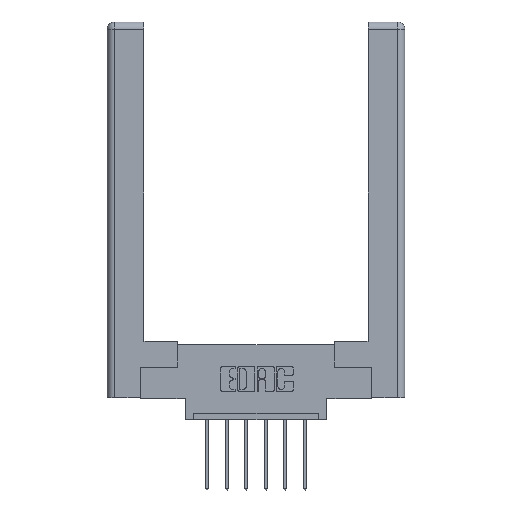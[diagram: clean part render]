
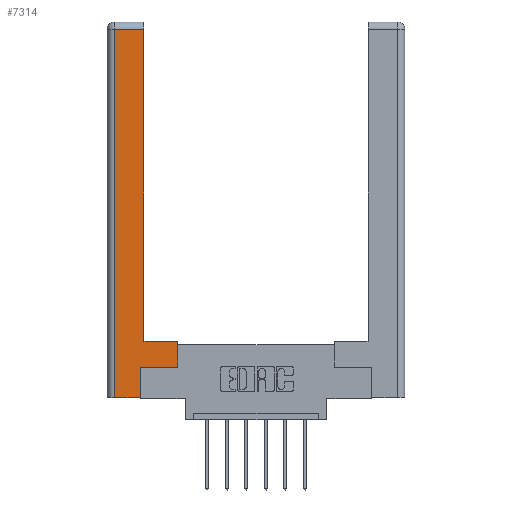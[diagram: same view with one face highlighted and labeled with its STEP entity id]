
A CAD part, top view. The second image highlights one B-rep face of the part: STEP entity #7314.
In plain terms, the highlighted planar face has unit normal (0, 0, 1).
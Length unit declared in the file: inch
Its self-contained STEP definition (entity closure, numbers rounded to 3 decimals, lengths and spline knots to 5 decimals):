
#93 = VECTOR ( 'NONE', #2105, 39.37008 ) ;
#392 = LINE ( 'NONE', #5843, #8719 ) ;
#776 = CARTESIAN_POINT ( 'NONE',  ( 0.265, 0., 0. ) ) ;
#900 = EDGE_CURVE ( 'NONE', #10897, #3169, #6829, .T. ) ;
#1043 = VERTEX_POINT ( 'NONE', #1053 ) ;
#1053 = CARTESIAN_POINT ( 'NONE',  ( 0.295, 0.45, 0. ) ) ;
#1106 = CARTESIAN_POINT ( 'NONE',  ( 0.295, 0.45, 0. ) ) ;
#1300 = LINE ( 'NONE', #4418, #10371 ) ;
#1707 = DIRECTION ( 'NONE',  ( 1., 0., 0. ) ) ;
#1950 = EDGE_CURVE ( 'NONE', #5651, #7742, #2416, .T. ) ;
#2014 = EDGE_LOOP ( 'NONE', ( #5442, #11224, #11188, #4874, #5051, #2156, #10419, #2401 ) ) ;
#2045 = DIRECTION ( 'NONE',  ( -1., 0., 0. ) ) ;
#2065 = CARTESIAN_POINT ( 'NONE',  ( 0.295, 3., 0. ) ) ;
#2073 = CARTESIAN_POINT ( 'NONE',  ( 0.565, 0.45, 0. ) ) ;
#2105 = DIRECTION ( 'NONE',  ( 0., 1., 0. ) ) ;
#2119 = AXIS2_PLACEMENT_3D ( 'NONE', #5973, #4154, #7884 ) ;
#2127 = EDGE_CURVE ( 'NONE', #2699, #1043, #5399, .T. ) ;
#2156 = ORIENTED_EDGE ( 'NONE', *, *, #8149, .T. ) ;
#2305 = VECTOR ( 'NONE', #10930, 39.37008 ) ;
#2401 = ORIENTED_EDGE ( 'NONE', *, *, #2127, .T. ) ;
#2416 = LINE ( 'NONE', #8247, #8305 ) ;
#2514 = VECTOR ( 'NONE', #1707, 39.37008 ) ;
#2685 = EDGE_CURVE ( 'NONE', #9537, #2699, #392, .T. ) ;
#2699 = VERTEX_POINT ( 'NONE', #2073 ) ;
#3102 = CARTESIAN_POINT ( 'NONE',  ( 0.265, 0., 0. ) ) ;
#3169 = VERTEX_POINT ( 'NONE', #3102 ) ;
#3200 = PLANE ( 'NONE',  #2119 ) ;
#3657 = CARTESIAN_POINT ( 'NONE',  ( 0.565, 0.245, 0. ) ) ;
#4154 = DIRECTION ( 'NONE',  ( 0., 0., -1. ) ) ;
#4418 = CARTESIAN_POINT ( 'NONE',  ( 0.0615, 0., 0. ) ) ;
#4874 = ORIENTED_EDGE ( 'NONE', *, *, #900, .T. ) ;
#5051 = ORIENTED_EDGE ( 'NONE', *, *, #8504, .T. ) ;
#5255 = FACE_OUTER_BOUND ( 'NONE', #2014, .T. ) ;
#5277 = VECTOR ( 'NONE', #7592, 39.37008 ) ;
#5399 = LINE ( 'NONE', #1106, #5695 ) ;
#5442 = ORIENTED_EDGE ( 'NONE', *, *, #10833, .T. ) ;
#5651 = VERTEX_POINT ( 'NONE', #9942 ) ;
#5695 = VECTOR ( 'NONE', #2045, 39.37008 ) ;
#5843 = CARTESIAN_POINT ( 'NONE',  ( 0.565, 0.45, 0. ) ) ;
#5973 = CARTESIAN_POINT ( 'NONE',  ( 0., 0., 0. ) ) ;
#6829 = LINE ( 'NONE', #776, #2514 ) ;
#6848 = CARTESIAN_POINT ( 'NONE',  ( 0.265, 0.245, 0. ) ) ;
#7193 = EDGE_CURVE ( 'NONE', #7742, #10897, #1300, .T. ) ;
#7253 = LINE ( 'NONE', #2065, #93 ) ;
#7309 = CARTESIAN_POINT ( 'NONE',  ( 0.565, 0.245, 0. ) ) ;
#7314 = ADVANCED_FACE ( 'NONE', ( #5255 ), #3200, .F. ) ;
#7465 = VERTEX_POINT ( 'NONE', #10876 ) ;
#7592 = DIRECTION ( 'NONE',  ( 0., 1., 0. ) ) ;
#7691 = CARTESIAN_POINT ( 'NONE',  ( 0.0615, 2.94, 0. ) ) ;
#7742 = VERTEX_POINT ( 'NONE', #7691 ) ;
#7884 = DIRECTION ( 'NONE',  ( -1., 0., 0. ) ) ;
#8065 = LINE ( 'NONE', #3657, #2305 ) ;
#8149 = EDGE_CURVE ( 'NONE', #7465, #9537, #8065, .T. ) ;
#8247 = CARTESIAN_POINT ( 'NONE',  ( 0.0615, 2.94, 0. ) ) ;
#8305 = VECTOR ( 'NONE', #11902, 39.37008 ) ;
#8332 = LINE ( 'NONE', #6848, #5277 ) ;
#8504 = EDGE_CURVE ( 'NONE', #3169, #7465, #8332, .T. ) ;
#8719 = VECTOR ( 'NONE', #11454, 39.37008 ) ;
#9537 = VERTEX_POINT ( 'NONE', #7309 ) ;
#9757 = CARTESIAN_POINT ( 'NONE',  ( 0.0615, 0., 0. ) ) ;
#9942 = CARTESIAN_POINT ( 'NONE',  ( 0.295, 2.94, 0. ) ) ;
#10371 = VECTOR ( 'NONE', #10798, 39.37008 ) ;
#10419 = ORIENTED_EDGE ( 'NONE', *, *, #2685, .T. ) ;
#10798 = DIRECTION ( 'NONE',  ( 0., -1., 0. ) ) ;
#10833 = EDGE_CURVE ( 'NONE', #1043, #5651, #7253, .T. ) ;
#10876 = CARTESIAN_POINT ( 'NONE',  ( 0.265, 0.245, 0. ) ) ;
#10897 = VERTEX_POINT ( 'NONE', #9757 ) ;
#10930 = DIRECTION ( 'NONE',  ( 1., 0., 0. ) ) ;
#11188 = ORIENTED_EDGE ( 'NONE', *, *, #7193, .T. ) ;
#11224 = ORIENTED_EDGE ( 'NONE', *, *, #1950, .T. ) ;
#11454 = DIRECTION ( 'NONE',  ( 0., 1., 0. ) ) ;
#11902 = DIRECTION ( 'NONE',  ( -1., 0., 0. ) ) ;
